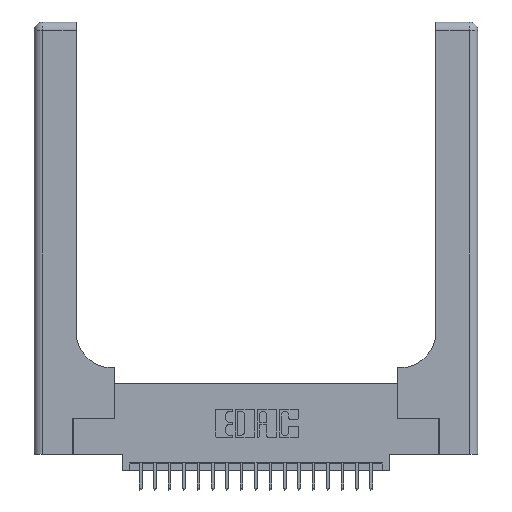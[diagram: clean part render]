
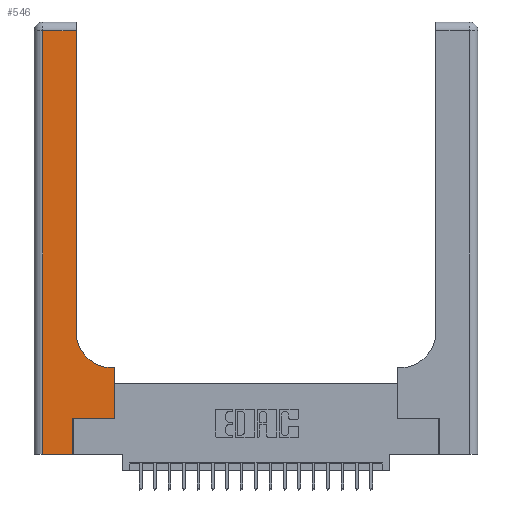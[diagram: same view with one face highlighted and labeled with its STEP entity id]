
A CAD part, top view. The second image highlights one B-rep face of the part: STEP entity #546.
In plain terms, the highlighted planar face has unit normal (0, 0, 1).
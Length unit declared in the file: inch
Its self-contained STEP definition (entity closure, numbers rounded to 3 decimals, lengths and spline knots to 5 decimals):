
#530 = AXIS2_PLACEMENT_3D ( 'NONE', #18511, #3173, #10216 ) ;
#546 = ADVANCED_FACE ( 'NONE', ( #13589 ), #11680, .F. ) ;
#783 = ORIENTED_EDGE ( 'NONE', *, *, #4323, .T. ) ;
#1181 = ORIENTED_EDGE ( 'NONE', *, *, #16086, .T. ) ;
#1241 = EDGE_CURVE ( 'NONE', #6481, #14914, #16429, .T. ) ;
#1475 = CARTESIAN_POINT ( 'NONE',  ( 0.269, 0., 0.37 ) ) ;
#2192 = ORIENTED_EDGE ( 'NONE', *, *, #1241, .T. ) ;
#2626 = VECTOR ( 'NONE', #10549, 39.37008 ) ;
#2787 = CARTESIAN_POINT ( 'NONE',  ( 0.2915, 0.6, 0.37 ) ) ;
#3173 = DIRECTION ( 'NONE',  ( 0., 0., -1. ) ) ;
#3302 = EDGE_LOOP ( 'NONE', ( #783, #6153, #8507, #4094, #2192, #4761, #18081, #18777, #1181 ) ) ;
#3728 = CARTESIAN_POINT ( 'NONE',  ( 0., 0., 0.37 ) ) ;
#3762 = CARTESIAN_POINT ( 'NONE',  ( 0.269, 0.25, 0.37 ) ) ;
#3833 = DIRECTION ( 'NONE',  ( 0., -1., 0. ) ) ;
#4094 = ORIENTED_EDGE ( 'NONE', *, *, #8879, .T. ) ;
#4105 = DIRECTION ( 'NONE',  ( 1., 0., 0. ) ) ;
#4119 = EDGE_CURVE ( 'NONE', #14914, #18974, #14399, .T. ) ;
#4140 = VERTEX_POINT ( 'NONE', #8784 ) ;
#4323 = EDGE_CURVE ( 'NONE', #4140, #11263, #9454, .T. ) ;
#4423 = CARTESIAN_POINT ( 'NONE',  ( 0.2915, 3., 0.37 ) ) ;
#4761 = ORIENTED_EDGE ( 'NONE', *, *, #4119, .T. ) ;
#4892 = VECTOR ( 'NONE', #16294, 39.37008 ) ;
#6153 = ORIENTED_EDGE ( 'NONE', *, *, #10781, .T. ) ;
#6465 = VERTEX_POINT ( 'NONE', #7743 ) ;
#6481 = VERTEX_POINT ( 'NONE', #1475 ) ;
#6755 = VERTEX_POINT ( 'NONE', #13569 ) ;
#7015 = VECTOR ( 'NONE', #10589, 39.37008 ) ;
#7019 = AXIS2_PLACEMENT_3D ( 'NONE', #19341, #20894, #4105 ) ;
#7344 = VECTOR ( 'NONE', #13181, 39.37008 ) ;
#7743 = CARTESIAN_POINT ( 'NONE',  ( 0.06, 2.94, 0.37 ) ) ;
#7925 = CARTESIAN_POINT ( 'NONE',  ( 0.5585, 0.25, 0.37 ) ) ;
#8284 = LINE ( 'NONE', #13669, #12650 ) ;
#8507 = ORIENTED_EDGE ( 'NONE', *, *, #19135, .T. ) ;
#8549 = VERTEX_POINT ( 'NONE', #21769 ) ;
#8656 = VECTOR ( 'NONE', #16455, 39.37008 ) ;
#8784 = CARTESIAN_POINT ( 'NONE',  ( 0.2915, 0.85, 0.37 ) ) ;
#8879 = EDGE_CURVE ( 'NONE', #21333, #6481, #19070, .T. ) ;
#9454 = LINE ( 'NONE', #4423, #4892 ) ;
#9493 = EDGE_CURVE ( 'NONE', #6755, #8549, #21489, .T. ) ;
#9752 = CARTESIAN_POINT ( 'NONE',  ( 0.06, 0., 0.37 ) ) ;
#9829 = DIRECTION ( 'NONE',  ( 0., 1., 0. ) ) ;
#10216 = DIRECTION ( 'NONE',  ( -1., 0., 0. ) ) ;
#10549 = DIRECTION ( 'NONE',  ( 1., 0., 0. ) ) ;
#10589 = DIRECTION ( 'NONE',  ( 1., 0., 0. ) ) ;
#10781 = EDGE_CURVE ( 'NONE', #11263, #6465, #8284, .T. ) ;
#11041 = VECTOR ( 'NONE', #3833, 39.37008 ) ;
#11242 = EDGE_CURVE ( 'NONE', #18974, #6755, #16453, .T. ) ;
#11263 = VERTEX_POINT ( 'NONE', #17118 ) ;
#11680 = PLANE ( 'NONE',  #530 ) ;
#12650 = VECTOR ( 'NONE', #20278, 39.37008 ) ;
#13181 = DIRECTION ( 'NONE',  ( 0., 1., 0. ) ) ;
#13256 = CARTESIAN_POINT ( 'NONE',  ( 0.5585, 0.25, 0.37 ) ) ;
#13569 = CARTESIAN_POINT ( 'NONE',  ( 0.5585, 0.6, 0.37 ) ) ;
#13589 = FACE_OUTER_BOUND ( 'NONE', #3302, .T. ) ;
#13669 = CARTESIAN_POINT ( 'NONE',  ( 0., 2.94, 0.37 ) ) ;
#14399 = LINE ( 'NONE', #3762, #7015 ) ;
#14846 = CARTESIAN_POINT ( 'NONE',  ( 0.269, 0.25, 0.37 ) ) ;
#14911 = CIRCLE ( 'NONE', #7019, 0.25 ) ;
#14914 = VERTEX_POINT ( 'NONE', #14846 ) ;
#15596 = LINE ( 'NONE', #20833, #11041 ) ;
#16086 = EDGE_CURVE ( 'NONE', #8549, #4140, #14911, .T. ) ;
#16294 = DIRECTION ( 'NONE',  ( 0., 1., 0. ) ) ;
#16429 = LINE ( 'NONE', #19896, #7344 ) ;
#16453 = LINE ( 'NONE', #7925, #18726 ) ;
#16455 = DIRECTION ( 'NONE',  ( -1., 0., 0. ) ) ;
#17118 = CARTESIAN_POINT ( 'NONE',  ( 0.2915, 2.94, 0.37 ) ) ;
#18081 = ORIENTED_EDGE ( 'NONE', *, *, #11242, .T. ) ;
#18511 = CARTESIAN_POINT ( 'NONE',  ( 0., 3., 0.37 ) ) ;
#18726 = VECTOR ( 'NONE', #9829, 39.37008 ) ;
#18777 = ORIENTED_EDGE ( 'NONE', *, *, #9493, .T. ) ;
#18974 = VERTEX_POINT ( 'NONE', #13256 ) ;
#19070 = LINE ( 'NONE', #3728, #2626 ) ;
#19135 = EDGE_CURVE ( 'NONE', #6465, #21333, #15596, .T. ) ;
#19341 = CARTESIAN_POINT ( 'NONE',  ( 0.5415, 0.85, 0.37 ) ) ;
#19896 = CARTESIAN_POINT ( 'NONE',  ( 0.269, 0., 0.37 ) ) ;
#20278 = DIRECTION ( 'NONE',  ( -1., 0., 0. ) ) ;
#20833 = CARTESIAN_POINT ( 'NONE',  ( 0.06, 3., 0.37 ) ) ;
#20894 = DIRECTION ( 'NONE',  ( 0., 0., -1. ) ) ;
#21333 = VERTEX_POINT ( 'NONE', #9752 ) ;
#21489 = LINE ( 'NONE', #2787, #8656 ) ;
#21769 = CARTESIAN_POINT ( 'NONE',  ( 0.5415, 0.6, 0.37 ) ) ;
